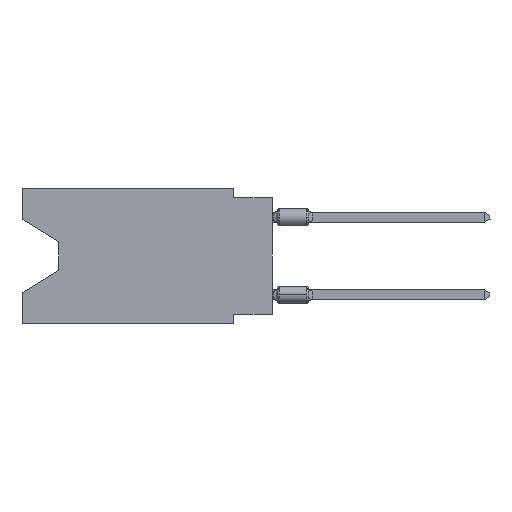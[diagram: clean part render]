
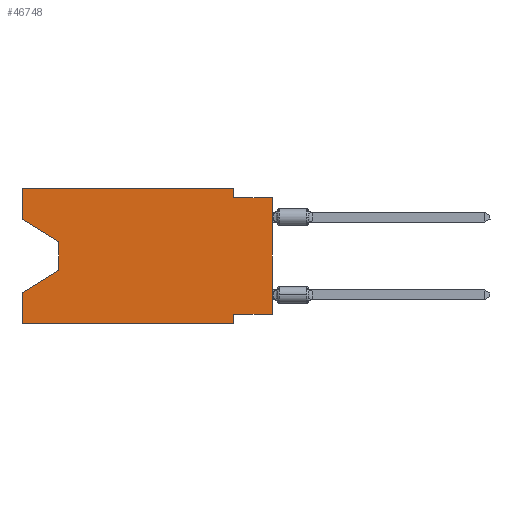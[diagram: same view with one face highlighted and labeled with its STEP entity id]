
A CAD part, left-side view. The second image highlights one B-rep face of the part: STEP entity #46748.
In plain terms, the highlighted planar face has unit normal (-1, 0, 0).
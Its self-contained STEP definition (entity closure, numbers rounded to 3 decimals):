
#786 = LINE ( 'NONE', #6380, #64117 ) ;
#1298 = ORIENTED_EDGE ( 'NONE', *, *, #23119, .T. ) ;
#1315 = CARTESIAN_POINT ( 'NONE',  ( 0., 16.383, -8.89 ) ) ;
#1463 = CARTESIAN_POINT ( 'NONE',  ( 0., 16.383, -2.038 ) ) ;
#2095 = VERTEX_POINT ( 'NONE', #41608 ) ;
#3306 = DIRECTION ( 'NONE',  ( 0., 1., 0. ) ) ;
#4681 = CARTESIAN_POINT ( 'NONE',  ( 0., 2.54, -0.635 ) ) ;
#4836 = EDGE_CURVE ( 'NONE', #2095, #63327, #73590, .T. ) ;
#5122 = VERTEX_POINT ( 'NONE', #31754 ) ;
#5578 = EDGE_CURVE ( 'NONE', #20725, #33955, #9132, .T. ) ;
#5771 = EDGE_CURVE ( 'NONE', #47863, #33955, #786, .T. ) ;
#6333 = LINE ( 'NONE', #67800, #61801 ) ;
#6380 = CARTESIAN_POINT ( 'NONE',  ( 0., 13.97, -5.385 ) ) ;
#6488 = DIRECTION ( 'NONE',  ( 0., 0., -1. ) ) ;
#7186 = DIRECTION ( 'NONE',  ( 0., -1., 0. ) ) ;
#9132 = LINE ( 'NONE', #66505, #56972 ) ;
#10804 = VERTEX_POINT ( 'NONE', #4681 ) ;
#10852 = DIRECTION ( 'NONE',  ( 0., 0., -1. ) ) ;
#11167 = ORIENTED_EDGE ( 'NONE', *, *, #12781, .F. ) ;
#12781 = EDGE_CURVE ( 'NONE', #10804, #63327, #53715, .T. ) ;
#13508 = CARTESIAN_POINT ( 'NONE',  ( 0., 0., -0.635 ) ) ;
#15797 = CARTESIAN_POINT ( 'NONE',  ( 0., 16.383, 0. ) ) ;
#16197 = ORIENTED_EDGE ( 'NONE', *, *, #22995, .F. ) ;
#16798 = LINE ( 'NONE', #61897, #21332 ) ;
#18503 = CARTESIAN_POINT ( 'NONE',  ( 0., 13.97, -3.505 ) ) ;
#18722 = LINE ( 'NONE', #41421, #56325 ) ;
#20365 = CARTESIAN_POINT ( 'NONE',  ( 0., 2.54, -8.255 ) ) ;
#20725 = VERTEX_POINT ( 'NONE', #1315 ) ;
#21332 = VECTOR ( 'NONE', #10852, 1000. ) ;
#21531 = AXIS2_PLACEMENT_3D ( 'NONE', #29189, #61992, #6488 ) ;
#22030 = CARTESIAN_POINT ( 'NONE',  ( 0., 13.97, -5.385 ) ) ;
#22995 = EDGE_CURVE ( 'NONE', #44981, #28716, #48317, .T. ) ;
#23119 = EDGE_CURVE ( 'NONE', #20725, #39591, #31199, .T. ) ;
#24615 = ORIENTED_EDGE ( 'NONE', *, *, #32824, .F. ) ;
#25618 = DIRECTION ( 'NONE',  ( 0., -1., 0. ) ) ;
#26491 = CARTESIAN_POINT ( 'NONE',  ( 0., 0., -0.635 ) ) ;
#26546 = EDGE_LOOP ( 'NONE', ( #59718, #58120, #65449, #38938, #1298, #29103, #24615, #67258, #11167, #39518, #42924, #16197 ) ) ;
#28343 = VECTOR ( 'NONE', #57910, 1000. ) ;
#28716 = VERTEX_POINT ( 'NONE', #15797 ) ;
#29040 = DIRECTION ( 'NONE',  ( 0., -0.855, -0.519 ) ) ;
#29103 = ORIENTED_EDGE ( 'NONE', *, *, #30359, .F. ) ;
#29189 = CARTESIAN_POINT ( 'NONE',  ( 0., 16.383, 0. ) ) ;
#30359 = EDGE_CURVE ( 'NONE', #70109, #39591, #16798, .T. ) ;
#30749 = DIRECTION ( 'NONE',  ( 0., 0., -1. ) ) ;
#31199 = LINE ( 'NONE', #53948, #54321 ) ;
#31754 = CARTESIAN_POINT ( 'NONE',  ( 0., 2.54, 0. ) ) ;
#31828 = DIRECTION ( 'NONE',  ( 0., 0., 1. ) ) ;
#32041 = VERTEX_POINT ( 'NONE', #67166 ) ;
#32314 = LINE ( 'NONE', #54700, #54222 ) ;
#32435 = VECTOR ( 'NONE', #30749, 1000. ) ;
#32824 = EDGE_CURVE ( 'NONE', #2095, #70109, #32314, .T. ) ;
#33955 = VERTEX_POINT ( 'NONE', #62226 ) ;
#35702 = CARTESIAN_POINT ( 'NONE',  ( 0., 16.383, 0. ) ) ;
#37424 = EDGE_CURVE ( 'NONE', #28716, #5122, #37994, .T. ) ;
#37994 = LINE ( 'NONE', #48797, #71587 ) ;
#38938 = ORIENTED_EDGE ( 'NONE', *, *, #5578, .F. ) ;
#39518 = ORIENTED_EDGE ( 'NONE', *, *, #61915, .F. ) ;
#39591 = VERTEX_POINT ( 'NONE', #62217 ) ;
#39879 = DIRECTION ( 'NONE',  ( 0., 0.855, -0.519 ) ) ;
#41421 = CARTESIAN_POINT ( 'NONE',  ( 0., 2.54, 0. ) ) ;
#41608 = CARTESIAN_POINT ( 'NONE',  ( 0., 0., -8.255 ) ) ;
#41932 = EDGE_CURVE ( 'NONE', #32041, #47863, #64315, .T. ) ;
#42008 = DIRECTION ( 'NONE',  ( 0., 0., 1. ) ) ;
#42924 = ORIENTED_EDGE ( 'NONE', *, *, #37424, .F. ) ;
#44819 = FACE_OUTER_BOUND ( 'NONE', #26546, .T. ) ;
#44981 = VERTEX_POINT ( 'NONE', #1463 ) ;
#46748 = ADVANCED_FACE ( 'NONE', ( #44819 ), #57505, .F. ) ;
#47863 = VERTEX_POINT ( 'NONE', #22030 ) ;
#48317 = LINE ( 'NONE', #35702, #55504 ) ;
#48797 = CARTESIAN_POINT ( 'NONE',  ( 0., 16.383, 0. ) ) ;
#49549 = DIRECTION ( 'NONE',  ( 0., -1., 0. ) ) ;
#53000 = DIRECTION ( 'NONE',  ( 0., 0., -1. ) ) ;
#53715 = LINE ( 'NONE', #13508, #60939 ) ;
#53948 = CARTESIAN_POINT ( 'NONE',  ( 0., 16.383, -8.89 ) ) ;
#54222 = VECTOR ( 'NONE', #3306, 1000. ) ;
#54321 = VECTOR ( 'NONE', #25618, 1000. ) ;
#54700 = CARTESIAN_POINT ( 'NONE',  ( 0., 0., -8.255 ) ) ;
#55504 = VECTOR ( 'NONE', #42008, 1000. ) ;
#56325 = VECTOR ( 'NONE', #53000, 1000. ) ;
#56972 = VECTOR ( 'NONE', #31828, 1000. ) ;
#57505 = PLANE ( 'NONE',  #21531 ) ;
#57910 = DIRECTION ( 'NONE',  ( 0., 0., 1. ) ) ;
#58120 = ORIENTED_EDGE ( 'NONE', *, *, #41932, .T. ) ;
#59029 = EDGE_CURVE ( 'NONE', #44981, #32041, #6333, .T. ) ;
#59718 = ORIENTED_EDGE ( 'NONE', *, *, #59029, .T. ) ;
#60939 = VECTOR ( 'NONE', #7186, 1000. ) ;
#61801 = VECTOR ( 'NONE', #29040, 1000. ) ;
#61897 = CARTESIAN_POINT ( 'NONE',  ( 0., 2.54, -8.89 ) ) ;
#61915 = EDGE_CURVE ( 'NONE', #5122, #10804, #18722, .T. ) ;
#61992 = DIRECTION ( 'NONE',  ( 1., 0., 0. ) ) ;
#62217 = CARTESIAN_POINT ( 'NONE',  ( 0., 2.54, -8.89 ) ) ;
#62226 = CARTESIAN_POINT ( 'NONE',  ( 0., 16.383, -6.852 ) ) ;
#63327 = VERTEX_POINT ( 'NONE', #26491 ) ;
#64117 = VECTOR ( 'NONE', #39879, 1000. ) ;
#64315 = LINE ( 'NONE', #18503, #32435 ) ;
#65449 = ORIENTED_EDGE ( 'NONE', *, *, #5771, .T. ) ;
#66505 = CARTESIAN_POINT ( 'NONE',  ( 0., 16.383, 0. ) ) ;
#67166 = CARTESIAN_POINT ( 'NONE',  ( 0., 13.97, -3.505 ) ) ;
#67258 = ORIENTED_EDGE ( 'NONE', *, *, #4836, .T. ) ;
#67800 = CARTESIAN_POINT ( 'NONE',  ( 0., 16.383, -2.038 ) ) ;
#68364 = CARTESIAN_POINT ( 'NONE',  ( 0., 0., 0. ) ) ;
#70109 = VERTEX_POINT ( 'NONE', #20365 ) ;
#71587 = VECTOR ( 'NONE', #49549, 1000. ) ;
#73590 = LINE ( 'NONE', #68364, #28343 ) ;
